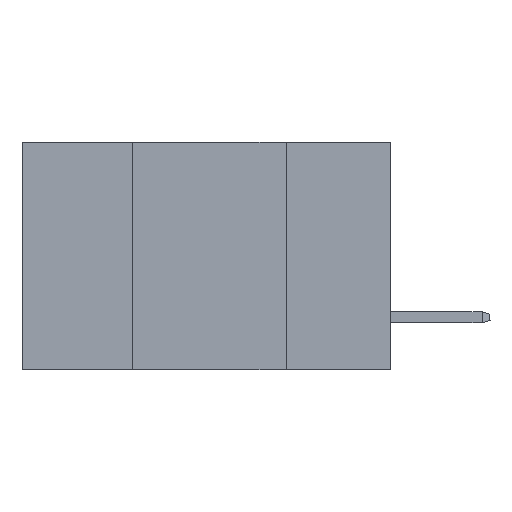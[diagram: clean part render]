
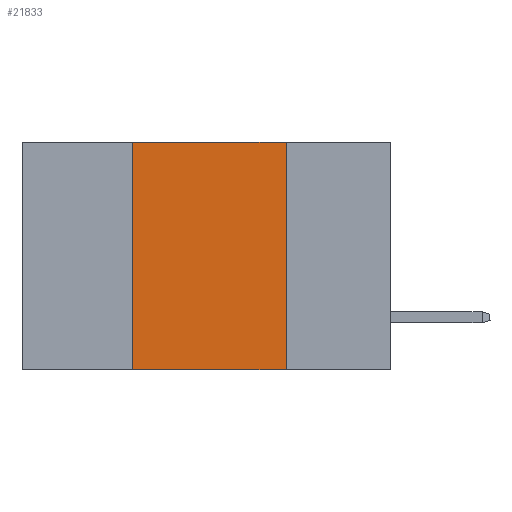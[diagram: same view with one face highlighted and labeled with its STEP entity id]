
A CAD part, left-side view. The second image highlights one B-rep face of the part: STEP entity #21833.
In plain terms, the highlighted planar face has unit normal (-1, 0, 0).
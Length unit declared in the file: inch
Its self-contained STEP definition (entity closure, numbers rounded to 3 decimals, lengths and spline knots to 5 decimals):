
#1062 = CARTESIAN_POINT ( 'NONE',  ( 0., 0.17, 0. ) ) ;
#1264 = EDGE_CURVE ( 'NONE', #4086, #15328, #28203, .T. ) ;
#1382 = VERTEX_POINT ( 'NONE', #5336 ) ;
#1671 = EDGE_CURVE ( 'NONE', #15328, #1382, #28517, .T. ) ;
#1926 = VERTEX_POINT ( 'NONE', #13196 ) ;
#3176 = VECTOR ( 'NONE', #28420, 39.37008 ) ;
#4086 = VERTEX_POINT ( 'NONE', #23390 ) ;
#4908 = CARTESIAN_POINT ( 'NONE',  ( 0., 0.6, 0. ) ) ;
#5336 = CARTESIAN_POINT ( 'NONE',  ( 0., 0.17, 0. ) ) ;
#6157 = VECTOR ( 'NONE', #11945, 39.37008 ) ;
#6284 = CARTESIAN_POINT ( 'NONE',  ( 0., 0.42, 0. ) ) ;
#6599 = ORIENTED_EDGE ( 'NONE', *, *, #1671, .F. ) ;
#6688 = VECTOR ( 'NONE', #12008, 39.37008 ) ;
#7531 = ORIENTED_EDGE ( 'NONE', *, *, #25762, .T. ) ;
#8139 = DIRECTION ( 'NONE',  ( 0., 0., -1. ) ) ;
#10368 = LINE ( 'NONE', #1062, #19092 ) ;
#11945 = DIRECTION ( 'NONE',  ( 0., 0., 1. ) ) ;
#12008 = DIRECTION ( 'NONE',  ( 0., -1., 0. ) ) ;
#13196 = CARTESIAN_POINT ( 'NONE',  ( 0., 0.17, -0.37 ) ) ;
#13772 = CARTESIAN_POINT ( 'NONE',  ( 0., 0.6, -0.37 ) ) ;
#14244 = DIRECTION ( 'NONE',  ( 1., 0., 0. ) ) ;
#14401 = CARTESIAN_POINT ( 'NONE',  ( 0., 0.6, 0. ) ) ;
#15328 = VERTEX_POINT ( 'NONE', #6284 ) ;
#16244 = ORIENTED_EDGE ( 'NONE', *, *, #1264, .F. ) ;
#16372 = EDGE_LOOP ( 'NONE', ( #24820, #6599, #16244, #7531 ) ) ;
#16570 = DIRECTION ( 'NONE',  ( 0., 0., -1. ) ) ;
#19092 = VECTOR ( 'NONE', #8139, 39.37008 ) ;
#19127 = PLANE ( 'NONE',  #26135 ) ;
#19744 = LINE ( 'NONE', #13772, #6688 ) ;
#21833 = ADVANCED_FACE ( 'NONE', ( #25015 ), #19127, .F. ) ;
#23390 = CARTESIAN_POINT ( 'NONE',  ( 0., 0.42, -0.37 ) ) ;
#23561 = EDGE_CURVE ( 'NONE', #1382, #1926, #10368, .T. ) ;
#24820 = ORIENTED_EDGE ( 'NONE', *, *, #23561, .F. ) ;
#25015 = FACE_OUTER_BOUND ( 'NONE', #16372, .T. ) ;
#25762 = EDGE_CURVE ( 'NONE', #4086, #1926, #19744, .T. ) ;
#25807 = CARTESIAN_POINT ( 'NONE',  ( 0., 0.42, 0. ) ) ;
#26135 = AXIS2_PLACEMENT_3D ( 'NONE', #4908, #14244, #16570 ) ;
#28203 = LINE ( 'NONE', #25807, #6157 ) ;
#28420 = DIRECTION ( 'NONE',  ( 0., -1., 0. ) ) ;
#28517 = LINE ( 'NONE', #14401, #3176 ) ;
